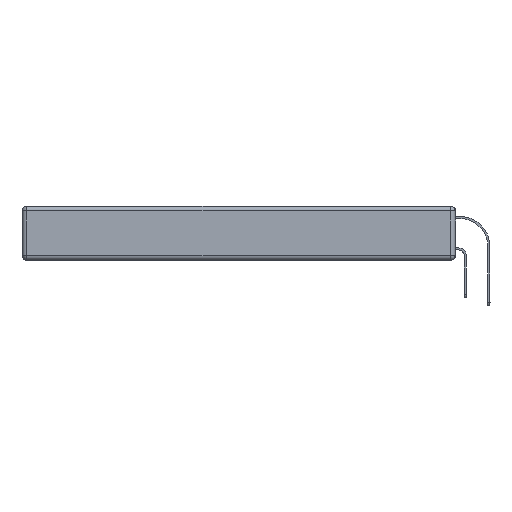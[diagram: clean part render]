
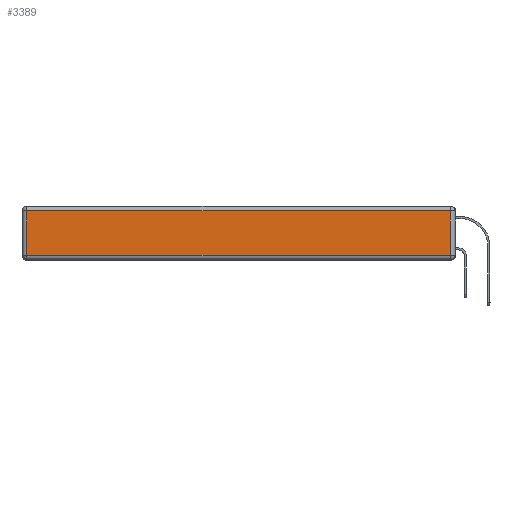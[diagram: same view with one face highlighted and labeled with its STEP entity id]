
A CAD part, left-side view. The second image highlights one B-rep face of the part: STEP entity #3389.
In plain terms, the highlighted planar face has unit normal (-1, 0, 0).
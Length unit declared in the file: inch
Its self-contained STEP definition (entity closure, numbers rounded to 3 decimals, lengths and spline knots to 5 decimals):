
#23 = LINE ( 'NONE', #9767, #5053 ) ;
#585 = ORIENTED_EDGE ( 'NONE', *, *, #23188, .T. ) ;
#600 = DIRECTION ( 'NONE',  ( 0., -1., 0. ) ) ;
#2590 = DIRECTION ( 'NONE',  ( -1., 0., 0. ) ) ;
#2720 = CARTESIAN_POINT ( 'NONE',  ( 0., 0., -0.343 ) ) ;
#3389 = ADVANCED_FACE ( 'NONE', ( #17976 ), #19363, .T. ) ;
#3643 = EDGE_LOOP ( 'NONE', ( #585, #18341, #18745, #4065 ) ) ;
#4065 = ORIENTED_EDGE ( 'NONE', *, *, #24403, .T. ) ;
#4371 = LINE ( 'NONE', #17994, #16455 ) ;
#5053 = VECTOR ( 'NONE', #22925, 39.37008 ) ;
#5071 = CARTESIAN_POINT ( 'NONE',  ( 0., 2.72, -0.313 ) ) ;
#6145 = DIRECTION ( 'NONE',  ( 0., 0., -1. ) ) ;
#6967 = EDGE_CURVE ( 'NONE', #18784, #8224, #11996, .T. ) ;
#8224 = VERTEX_POINT ( 'NONE', #13906 ) ;
#9767 = CARTESIAN_POINT ( 'NONE',  ( 0., 2.75, -0.03 ) ) ;
#9997 = LINE ( 'NONE', #11505, #10089 ) ;
#10030 = VERTEX_POINT ( 'NONE', #11558 ) ;
#10089 = VECTOR ( 'NONE', #6145, 39.37008 ) ;
#11505 = CARTESIAN_POINT ( 'NONE',  ( 0., 2.72, -0.343 ) ) ;
#11558 = CARTESIAN_POINT ( 'NONE',  ( 0., 2.72, -0.03 ) ) ;
#11996 = LINE ( 'NONE', #14110, #14374 ) ;
#12208 = DIRECTION ( 'NONE',  ( 0., 0., 1. ) ) ;
#12596 = AXIS2_PLACEMENT_3D ( 'NONE', #2720, #2590, #12208 ) ;
#12849 = EDGE_CURVE ( 'NONE', #8224, #10030, #23, .T. ) ;
#13906 = CARTESIAN_POINT ( 'NONE',  ( 0., 0.03, -0.03 ) ) ;
#14110 = CARTESIAN_POINT ( 'NONE',  ( 0., 0.03, -0.343 ) ) ;
#14374 = VECTOR ( 'NONE', #21648, 39.37008 ) ;
#16455 = VECTOR ( 'NONE', #600, 39.37008 ) ;
#17976 = FACE_OUTER_BOUND ( 'NONE', #3643, .T. ) ;
#17994 = CARTESIAN_POINT ( 'NONE',  ( 0., 0., -0.313 ) ) ;
#18341 = ORIENTED_EDGE ( 'NONE', *, *, #6967, .T. ) ;
#18745 = ORIENTED_EDGE ( 'NONE', *, *, #12849, .T. ) ;
#18784 = VERTEX_POINT ( 'NONE', #22675 ) ;
#19363 = PLANE ( 'NONE',  #12596 ) ;
#21648 = DIRECTION ( 'NONE',  ( 0., 0., 1. ) ) ;
#22675 = CARTESIAN_POINT ( 'NONE',  ( 0., 0.03, -0.313 ) ) ;
#22925 = DIRECTION ( 'NONE',  ( 0., 1., 0. ) ) ;
#23188 = EDGE_CURVE ( 'NONE', #23624, #18784, #4371, .T. ) ;
#23624 = VERTEX_POINT ( 'NONE', #5071 ) ;
#24403 = EDGE_CURVE ( 'NONE', #10030, #23624, #9997, .T. ) ;
